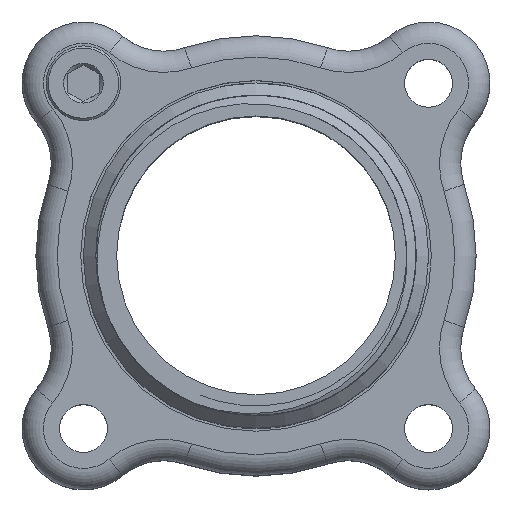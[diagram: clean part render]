
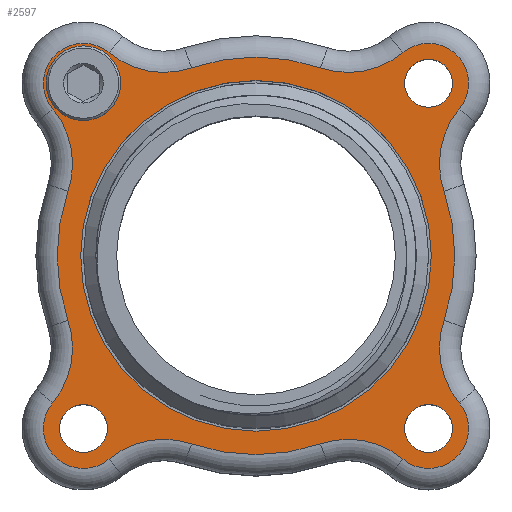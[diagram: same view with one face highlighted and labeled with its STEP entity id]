
A CAD part, top view. The second image highlights one B-rep face of the part: STEP entity #2597.
In plain terms, the highlighted planar face has unit normal (0, 0, 1).
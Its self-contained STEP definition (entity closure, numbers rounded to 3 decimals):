
#121=FACE_BOUND('',#417,.T.);
#122=FACE_BOUND('',#418,.T.);
#123=FACE_BOUND('',#419,.T.);
#124=FACE_BOUND('',#420,.T.);
#125=FACE_BOUND('',#421,.T.);
#159=PLANE('',#2905);
#248=FACE_OUTER_BOUND('',#416,.T.);
#416=EDGE_LOOP('',(#1984,#1985,#1986,#1987,#1988,#1989,#1990,#1991,#1992,
#1993,#1994,#1995,#1996,#1997,#1998,#1999));
#417=EDGE_LOOP('',(#2000));
#418=EDGE_LOOP('',(#2001));
#419=EDGE_LOOP('',(#2002));
#420=EDGE_LOOP('',(#2003));
#421=EDGE_LOOP('',(#2004));
#552=CIRCLE('',#2827,8.);
#557=CIRCLE('',#2833,18.65);
#560=CIRCLE('',#2837,8.);
#563=CIRCLE('',#2841,3.75);
#566=CIRCLE('',#2845,8.);
#569=CIRCLE('',#2849,18.65);
#572=CIRCLE('',#2853,8.);
#575=CIRCLE('',#2857,3.75);
#578=CIRCLE('',#2861,8.);
#581=CIRCLE('',#2865,18.65);
#584=CIRCLE('',#2869,8.);
#587=CIRCLE('',#2873,3.75);
#590=CIRCLE('',#2877,8.);
#593=CIRCLE('',#2881,18.65);
#596=CIRCLE('',#2885,8.);
#597=CIRCLE('',#2887,3.75);
#607=CIRCLE('',#2906,2.25);
#608=CIRCLE('',#2907,16.45);
#609=CIRCLE('',#2908,2.25);
#610=CIRCLE('',#2909,2.25);
#611=CIRCLE('',#2910,2.25);
#1075=VERTEX_POINT('',#6255);
#1076=VERTEX_POINT('',#6257);
#1078=VERTEX_POINT('',#6263);
#1080=VERTEX_POINT('',#6269);
#1082=VERTEX_POINT('',#6275);
#1084=VERTEX_POINT('',#6281);
#1086=VERTEX_POINT('',#6287);
#1088=VERTEX_POINT('',#6293);
#1090=VERTEX_POINT('',#6299);
#1092=VERTEX_POINT('',#6305);
#1094=VERTEX_POINT('',#6311);
#1096=VERTEX_POINT('',#6317);
#1098=VERTEX_POINT('',#6323);
#1100=VERTEX_POINT('',#6329);
#1102=VERTEX_POINT('',#6335);
#1104=VERTEX_POINT('',#6341);
#1115=VERTEX_POINT('',#6384);
#1116=VERTEX_POINT('',#6386);
#1117=VERTEX_POINT('',#6388);
#1118=VERTEX_POINT('',#6390);
#1119=VERTEX_POINT('',#6392);
#1372=EDGE_CURVE('',#1075,#1076,#552,.T.);
#1377=EDGE_CURVE('',#1076,#1078,#557,.T.);
#1380=EDGE_CURVE('',#1078,#1080,#560,.T.);
#1383=EDGE_CURVE('',#1080,#1082,#563,.T.);
#1386=EDGE_CURVE('',#1082,#1084,#566,.T.);
#1389=EDGE_CURVE('',#1084,#1086,#569,.T.);
#1392=EDGE_CURVE('',#1086,#1088,#572,.T.);
#1395=EDGE_CURVE('',#1088,#1090,#575,.T.);
#1398=EDGE_CURVE('',#1090,#1092,#578,.T.);
#1401=EDGE_CURVE('',#1092,#1094,#581,.T.);
#1404=EDGE_CURVE('',#1094,#1096,#584,.T.);
#1407=EDGE_CURVE('',#1096,#1098,#587,.T.);
#1410=EDGE_CURVE('',#1098,#1100,#590,.T.);
#1413=EDGE_CURVE('',#1100,#1102,#593,.T.);
#1416=EDGE_CURVE('',#1102,#1104,#596,.T.);
#1417=EDGE_CURVE('',#1104,#1075,#597,.T.);
#1436=EDGE_CURVE('',#1115,#1115,#607,.T.);
#1437=EDGE_CURVE('',#1116,#1116,#608,.F.);
#1438=EDGE_CURVE('',#1117,#1117,#609,.T.);
#1439=EDGE_CURVE('',#1118,#1118,#610,.T.);
#1440=EDGE_CURVE('',#1119,#1119,#611,.T.);
#1984=ORIENTED_EDGE('',*,*,#1372,.F.);
#1985=ORIENTED_EDGE('',*,*,#1417,.F.);
#1986=ORIENTED_EDGE('',*,*,#1416,.F.);
#1987=ORIENTED_EDGE('',*,*,#1413,.F.);
#1988=ORIENTED_EDGE('',*,*,#1410,.F.);
#1989=ORIENTED_EDGE('',*,*,#1407,.F.);
#1990=ORIENTED_EDGE('',*,*,#1404,.F.);
#1991=ORIENTED_EDGE('',*,*,#1401,.F.);
#1992=ORIENTED_EDGE('',*,*,#1398,.F.);
#1993=ORIENTED_EDGE('',*,*,#1395,.F.);
#1994=ORIENTED_EDGE('',*,*,#1392,.F.);
#1995=ORIENTED_EDGE('',*,*,#1389,.F.);
#1996=ORIENTED_EDGE('',*,*,#1386,.F.);
#1997=ORIENTED_EDGE('',*,*,#1383,.F.);
#1998=ORIENTED_EDGE('',*,*,#1380,.F.);
#1999=ORIENTED_EDGE('',*,*,#1377,.F.);
#2000=ORIENTED_EDGE('',*,*,#1436,.T.);
#2001=ORIENTED_EDGE('',*,*,#1437,.T.);
#2002=ORIENTED_EDGE('',*,*,#1438,.T.);
#2003=ORIENTED_EDGE('',*,*,#1439,.T.);
#2004=ORIENTED_EDGE('',*,*,#1440,.T.);
#2597=ADVANCED_FACE('',(#248,#121,#122,#123,#124,#125),#159,.T.);
#2827=AXIS2_PLACEMENT_3D('',#6258,#3314,#3315);
#2833=AXIS2_PLACEMENT_3D('',#6267,#3326,#3327);
#2837=AXIS2_PLACEMENT_3D('',#6273,#3334,#3335);
#2841=AXIS2_PLACEMENT_3D('',#6279,#3342,#3343);
#2845=AXIS2_PLACEMENT_3D('',#6285,#3350,#3351);
#2849=AXIS2_PLACEMENT_3D('',#6291,#3358,#3359);
#2853=AXIS2_PLACEMENT_3D('',#6297,#3366,#3367);
#2857=AXIS2_PLACEMENT_3D('',#6303,#3374,#3375);
#2861=AXIS2_PLACEMENT_3D('',#6309,#3382,#3383);
#2865=AXIS2_PLACEMENT_3D('',#6315,#3390,#3391);
#2869=AXIS2_PLACEMENT_3D('',#6321,#3398,#3399);
#2873=AXIS2_PLACEMENT_3D('',#6327,#3406,#3407);
#2877=AXIS2_PLACEMENT_3D('',#6333,#3414,#3415);
#2881=AXIS2_PLACEMENT_3D('',#6339,#3422,#3423);
#2885=AXIS2_PLACEMENT_3D('',#6345,#3430,#3431);
#2887=AXIS2_PLACEMENT_3D('',#6347,#3434,#3435);
#2905=AXIS2_PLACEMENT_3D('',#6383,#3479,#3480);
#2906=AXIS2_PLACEMENT_3D('',#6385,#3481,#3482);
#2907=AXIS2_PLACEMENT_3D('',#6387,#3483,#3484);
#2908=AXIS2_PLACEMENT_3D('',#6389,#3485,#3486);
#2909=AXIS2_PLACEMENT_3D('',#6391,#3487,#3488);
#2910=AXIS2_PLACEMENT_3D('',#6393,#3489,#3490);
#3314=DIRECTION('center_axis',(0.,0.,1.));
#3315=DIRECTION('ref_axis',(0.182,0.983,0.));
#3326=DIRECTION('center_axis',(0.,0.,-1.));
#3327=DIRECTION('ref_axis',(0.,-1.,0.));
#3334=DIRECTION('center_axis',(0.,0.,1.));
#3335=DIRECTION('ref_axis',(-0.182,0.983,0.));
#3342=DIRECTION('center_axis',(0.,0.,-1.));
#3343=DIRECTION('ref_axis',(-0.707,-0.707,0.));
#3350=DIRECTION('center_axis',(0.,0.,1.));
#3351=DIRECTION('ref_axis',(0.983,-0.182,0.));
#3358=DIRECTION('center_axis',(0.,0.,-1.));
#3359=DIRECTION('ref_axis',(-1.,0.,0.));
#3366=DIRECTION('center_axis',(0.,0.,1.));
#3367=DIRECTION('ref_axis',(0.983,0.182,0.));
#3374=DIRECTION('center_axis',(0.,0.,-1.));
#3375=DIRECTION('ref_axis',(-0.707,0.707,0.));
#3382=DIRECTION('center_axis',(0.,0.,1.));
#3383=DIRECTION('ref_axis',(-0.182,-0.983,0.));
#3390=DIRECTION('center_axis',(0.,0.,-1.));
#3391=DIRECTION('ref_axis',(0.,1.,0.));
#3398=DIRECTION('center_axis',(0.,0.,1.));
#3399=DIRECTION('ref_axis',(0.182,-0.983,0.));
#3406=DIRECTION('center_axis',(0.,0.,-1.));
#3407=DIRECTION('ref_axis',(0.707,0.707,0.));
#3414=DIRECTION('center_axis',(0.,0.,1.));
#3415=DIRECTION('ref_axis',(-0.983,0.182,0.));
#3422=DIRECTION('center_axis',(0.,0.,-1.));
#3423=DIRECTION('ref_axis',(1.,0.,0.));
#3430=DIRECTION('center_axis',(0.,0.,1.));
#3431=DIRECTION('ref_axis',(-0.983,-0.182,0.));
#3434=DIRECTION('center_axis',(0.,0.,-1.));
#3435=DIRECTION('ref_axis',(0.707,-0.707,0.));
#3479=DIRECTION('center_axis',(0.,0.,1.));
#3480=DIRECTION('ref_axis',(-1.,0.,0.));
#3481=DIRECTION('center_axis',(0.,0.,-1.));
#3482=DIRECTION('ref_axis',(1.,0.,0.));
#3483=DIRECTION('center_axis',(0.,0.,1.));
#3484=DIRECTION('ref_axis',(-1.,0.,0.));
#3485=DIRECTION('center_axis',(0.,0.,-1.));
#3486=DIRECTION('ref_axis',(1.,0.,0.));
#3487=DIRECTION('center_axis',(0.,0.,-1.));
#3488=DIRECTION('ref_axis',(1.,0.,0.));
#3489=DIRECTION('center_axis',(0.,0.,-1.));
#3490=DIRECTION('ref_axis',(1.,0.,0.));
#6255=CARTESIAN_POINT('',(13.787,-19.069,10.2));
#6257=CARTESIAN_POINT('',(6.056,-17.639,10.2));
#6258=CARTESIAN_POINT('Origin',(8.654,-25.206,10.2));
#6263=CARTESIAN_POINT('',(-6.056,-17.639,10.2));
#6267=CARTESIAN_POINT('Origin',(0.,0.,10.2));
#6269=CARTESIAN_POINT('',(-13.787,-19.069,10.2));
#6273=CARTESIAN_POINT('Origin',(-8.654,-25.206,10.2));
#6275=CARTESIAN_POINT('',(-19.069,-13.787,10.2));
#6279=CARTESIAN_POINT('Origin',(-16.193,-16.193,10.2));
#6281=CARTESIAN_POINT('',(-17.639,-6.056,10.2));
#6285=CARTESIAN_POINT('Origin',(-25.206,-8.654,10.2));
#6287=CARTESIAN_POINT('',(-17.639,6.056,10.2));
#6291=CARTESIAN_POINT('Origin',(0.,0.,10.2));
#6293=CARTESIAN_POINT('',(-19.069,13.787,10.2));
#6297=CARTESIAN_POINT('Origin',(-25.206,8.654,10.2));
#6299=CARTESIAN_POINT('',(-13.787,19.069,10.2));
#6303=CARTESIAN_POINT('Origin',(-16.193,16.193,10.2));
#6305=CARTESIAN_POINT('',(-6.056,17.639,10.2));
#6309=CARTESIAN_POINT('Origin',(-8.654,25.206,10.2));
#6311=CARTESIAN_POINT('',(6.056,17.639,10.2));
#6315=CARTESIAN_POINT('Origin',(0.,0.,10.2));
#6317=CARTESIAN_POINT('',(13.787,19.069,10.2));
#6321=CARTESIAN_POINT('Origin',(8.654,25.206,10.2));
#6323=CARTESIAN_POINT('',(19.069,13.787,10.2));
#6327=CARTESIAN_POINT('Origin',(16.193,16.193,10.2));
#6329=CARTESIAN_POINT('',(17.639,6.056,10.2));
#6333=CARTESIAN_POINT('Origin',(25.206,8.654,10.2));
#6335=CARTESIAN_POINT('',(17.639,-6.056,10.2));
#6339=CARTESIAN_POINT('Origin',(0.,0.,10.2));
#6341=CARTESIAN_POINT('',(19.069,-13.787,10.2));
#6345=CARTESIAN_POINT('Origin',(25.206,-8.654,10.2));
#6347=CARTESIAN_POINT('Origin',(16.193,-16.193,10.2));
#6383=CARTESIAN_POINT('Origin',(0.,0.,10.2));
#6384=CARTESIAN_POINT('',(13.943,-16.193,10.2));
#6385=CARTESIAN_POINT('Origin',(16.193,-16.193,10.2));
#6386=CARTESIAN_POINT('',(16.45,0.,10.2));
#6387=CARTESIAN_POINT('Origin',(0.,0.,10.2));
#6388=CARTESIAN_POINT('',(-18.443,16.193,10.2));
#6389=CARTESIAN_POINT('Origin',(-16.193,16.193,10.2));
#6390=CARTESIAN_POINT('',(-18.443,-16.193,10.2));
#6391=CARTESIAN_POINT('Origin',(-16.193,-16.193,10.2));
#6392=CARTESIAN_POINT('',(13.943,16.193,10.2));
#6393=CARTESIAN_POINT('Origin',(16.193,16.193,10.2));
